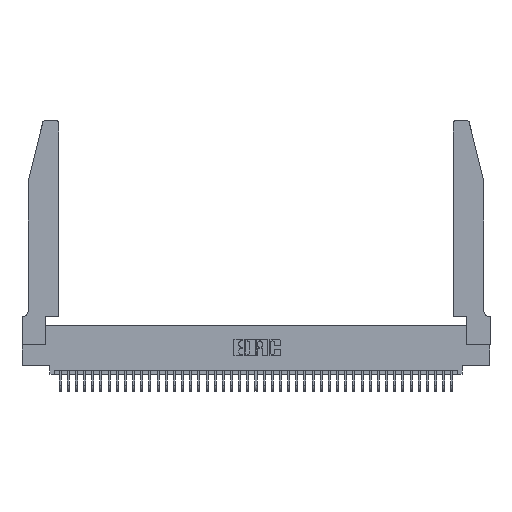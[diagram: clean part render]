
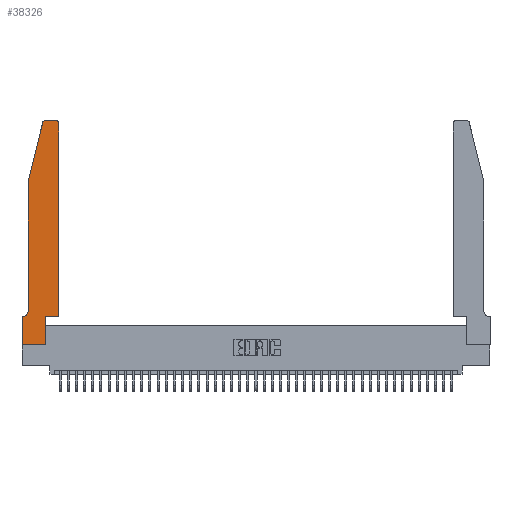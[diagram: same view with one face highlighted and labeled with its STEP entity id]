
A CAD part, top view. The second image highlights one B-rep face of the part: STEP entity #38326.
In plain terms, the highlighted planar face has unit normal (0, 0, 1).
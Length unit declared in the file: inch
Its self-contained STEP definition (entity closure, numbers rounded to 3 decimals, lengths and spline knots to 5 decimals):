
#499 = CARTESIAN_POINT ( 'NONE',  ( 0.0755, 2., 0.37 ) ) ;
#517 = ORIENTED_EDGE ( 'NONE', *, *, #40792, .T. ) ;
#710 = CARTESIAN_POINT ( 'NONE',  ( 0., 0., 0.37 ) ) ;
#1684 = DIRECTION ( 'NONE',  ( -1., 0., 0. ) ) ;
#2917 = DIRECTION ( 'NONE',  ( 0., 0., 1. ) ) ;
#3287 = ORIENTED_EDGE ( 'NONE', *, *, #14220, .T. ) ;
#3686 = EDGE_LOOP ( 'NONE', ( #32409, #3287, #17479, #41431, #13650, #40261, #14280, #517, #28158, #6649, #18911, #6212 ) ) ;
#3842 = DIRECTION ( 'NONE',  ( 1., 0., 0. ) ) ;
#5284 = DIRECTION ( 'NONE',  ( 0., 1., 0. ) ) ;
#5903 = DIRECTION ( 'NONE',  ( 1., 0., 0. ) ) ;
#6018 = CARTESIAN_POINT ( 'NONE',  ( 0.0055, 0.35, 0.37 ) ) ;
#6061 = LINE ( 'NONE', #29420, #16135 ) ;
#6212 = ORIENTED_EDGE ( 'NONE', *, *, #42006, .T. ) ;
#6551 = LINE ( 'NONE', #43830, #17145 ) ;
#6649 = ORIENTED_EDGE ( 'NONE', *, *, #24339, .T. ) ;
#7340 = VERTEX_POINT ( 'NONE', #499 ) ;
#8129 = DIRECTION ( 'NONE',  ( -0.239, -0.971, 0. ) ) ;
#8304 = CARTESIAN_POINT ( 'NONE',  ( 0.0055, 0.42, 0.37 ) ) ;
#8893 = DIRECTION ( 'NONE',  ( 0., -1., 0. ) ) ;
#9343 = CARTESIAN_POINT ( 'NONE',  ( 0., 0., 0.37 ) ) ;
#9999 = AXIS2_PLACEMENT_3D ( 'NONE', #41451, #17824, #31255 ) ;
#10471 = LINE ( 'NONE', #9343, #42308 ) ;
#11280 = EDGE_CURVE ( 'NONE', #39350, #13255, #10471, .T. ) ;
#11479 = FACE_OUTER_BOUND ( 'NONE', #3686, .T. ) ;
#13255 = VERTEX_POINT ( 'NONE', #710 ) ;
#13650 = ORIENTED_EDGE ( 'NONE', *, *, #29005, .T. ) ;
#14220 = EDGE_CURVE ( 'NONE', #36753, #18155, #42134, .T. ) ;
#14280 = ORIENTED_EDGE ( 'NONE', *, *, #11280, .T. ) ;
#14797 = CARTESIAN_POINT ( 'NONE',  ( 0.284, 2.75, 0.37 ) ) ;
#15051 = LINE ( 'NONE', #43553, #32064 ) ;
#15242 = DIRECTION ( 'NONE',  ( 0., 0., -1. ) ) ;
#15613 = EDGE_CURVE ( 'NONE', #42889, #36007, #6061, .T. ) ;
#16135 = VECTOR ( 'NONE', #5284, 39.37008 ) ;
#16411 = CARTESIAN_POINT ( 'NONE',  ( 0.4505, 0.35, 0.37 ) ) ;
#17145 = VECTOR ( 'NONE', #33601, 39.37008 ) ;
#17454 = LINE ( 'NONE', #43038, #37149 ) ;
#17479 = ORIENTED_EDGE ( 'NONE', *, *, #18498, .T. ) ;
#17507 = CARTESIAN_POINT ( 'NONE',  ( 0.2865, 0., 0.37 ) ) ;
#17824 = DIRECTION ( 'NONE',  ( 0., 0., 1. ) ) ;
#18155 = VERTEX_POINT ( 'NONE', #26859 ) ;
#18498 = EDGE_CURVE ( 'NONE', #18155, #7340, #31305, .T. ) ;
#18834 = CARTESIAN_POINT ( 'NONE',  ( 0.4205, 2.72, 0.37 ) ) ;
#18911 = ORIENTED_EDGE ( 'NONE', *, *, #15613, .T. ) ;
#20234 = VERTEX_POINT ( 'NONE', #27464 ) ;
#20630 = DIRECTION ( 'NONE',  ( 1., 0., 0. ) ) ;
#21349 = LINE ( 'NONE', #31890, #43174 ) ;
#21889 = VERTEX_POINT ( 'NONE', #35162 ) ;
#22572 = CARTESIAN_POINT ( 'NONE',  ( 0.0755, 0.35, 0.37 ) ) ;
#23639 = DIRECTION ( 'NONE',  ( 0., 0., 1. ) ) ;
#24339 = EDGE_CURVE ( 'NONE', #21889, #42889, #37945, .T. ) ;
#24898 = EDGE_CURVE ( 'NONE', #20234, #36753, #15051, .T. ) ;
#26571 = AXIS2_PLACEMENT_3D ( 'NONE', #18834, #2917, #36954 ) ;
#26623 = VERTEX_POINT ( 'NONE', #17507 ) ;
#26859 = CARTESIAN_POINT ( 'NONE',  ( 0.25487, 2.72718, 0.37 ) ) ;
#27119 = VECTOR ( 'NONE', #8129, 39.37008 ) ;
#27448 = EDGE_CURVE ( 'NONE', #31205, #39350, #36684, .T. ) ;
#27464 = CARTESIAN_POINT ( 'NONE',  ( 0.4205, 2.75, 0.37 ) ) ;
#28016 = EDGE_CURVE ( 'NONE', #7340, #35905, #21349, .T. ) ;
#28158 = ORIENTED_EDGE ( 'NONE', *, *, #39593, .T. ) ;
#29005 = EDGE_CURVE ( 'NONE', #35905, #31205, #33258, .T. ) ;
#29420 = CARTESIAN_POINT ( 'NONE',  ( 0.4505, 0.35, 0.37 ) ) ;
#30227 = DIRECTION ( 'NONE',  ( -1., 0., 0. ) ) ;
#31205 = VERTEX_POINT ( 'NONE', #6018 ) ;
#31255 = DIRECTION ( 'NONE',  ( 1., 0., 0. ) ) ;
#31305 = LINE ( 'NONE', #39188, #27119 ) ;
#31890 = CARTESIAN_POINT ( 'NONE',  ( 0.0755, 2., 0.37 ) ) ;
#31963 = CARTESIAN_POINT ( 'NONE',  ( 0.4505, 2.72, 0.37 ) ) ;
#31996 = CARTESIAN_POINT ( 'NONE',  ( 0., 0.35, 0.37 ) ) ;
#32064 = VECTOR ( 'NONE', #30227, 39.37008 ) ;
#32409 = ORIENTED_EDGE ( 'NONE', *, *, #24898, .T. ) ;
#33258 = CIRCLE ( 'NONE', #38742, 0.07 ) ;
#33601 = DIRECTION ( 'NONE',  ( 0., 1., 0. ) ) ;
#34276 = PLANE ( 'NONE',  #43488 ) ;
#34323 = CARTESIAN_POINT ( 'NONE',  ( 0.4505, 0.35, 0.37 ) ) ;
#34508 = CIRCLE ( 'NONE', #26571, 0.03 ) ;
#35162 = CARTESIAN_POINT ( 'NONE',  ( 0.2865, 0.35, 0.37 ) ) ;
#35905 = VERTEX_POINT ( 'NONE', #41267 ) ;
#36007 = VERTEX_POINT ( 'NONE', #31963 ) ;
#36684 = LINE ( 'NONE', #22572, #38778 ) ;
#36753 = VERTEX_POINT ( 'NONE', #14797 ) ;
#36954 = DIRECTION ( 'NONE',  ( 1., 0., 0. ) ) ;
#37149 = VECTOR ( 'NONE', #5903, 39.37008 ) ;
#37945 = LINE ( 'NONE', #34323, #41653 ) ;
#37950 = DIRECTION ( 'NONE',  ( 0., -1., 0. ) ) ;
#38326 = ADVANCED_FACE ( 'NONE', ( #11479 ), #34276, .T. ) ;
#38742 = AXIS2_PLACEMENT_3D ( 'NONE', #8304, #15242, #42449 ) ;
#38778 = VECTOR ( 'NONE', #1684, 39.37008 ) ;
#39188 = CARTESIAN_POINT ( 'NONE',  ( 0.0755, 2., 0.37 ) ) ;
#39350 = VERTEX_POINT ( 'NONE', #31996 ) ;
#39593 = EDGE_CURVE ( 'NONE', #26623, #21889, #6551, .T. ) ;
#40261 = ORIENTED_EDGE ( 'NONE', *, *, #27448, .T. ) ;
#40792 = EDGE_CURVE ( 'NONE', #13255, #26623, #17454, .T. ) ;
#41267 = CARTESIAN_POINT ( 'NONE',  ( 0.0755, 0.42, 0.37 ) ) ;
#41431 = ORIENTED_EDGE ( 'NONE', *, *, #28016, .T. ) ;
#41451 = CARTESIAN_POINT ( 'NONE',  ( 0.284, 2.72, 0.37 ) ) ;
#41653 = VECTOR ( 'NONE', #3842, 39.37008 ) ;
#42006 = EDGE_CURVE ( 'NONE', #36007, #20234, #34508, .T. ) ;
#42134 = CIRCLE ( 'NONE', #9999, 0.03 ) ;
#42308 = VECTOR ( 'NONE', #8893, 39.37008 ) ;
#42449 = DIRECTION ( 'NONE',  ( -1., 0., 0. ) ) ;
#42889 = VERTEX_POINT ( 'NONE', #16411 ) ;
#42992 = CARTESIAN_POINT ( 'NONE',  ( 0., 0.35, 0.37 ) ) ;
#43038 = CARTESIAN_POINT ( 'NONE',  ( 0., 0., 0.37 ) ) ;
#43174 = VECTOR ( 'NONE', #37950, 39.37008 ) ;
#43488 = AXIS2_PLACEMENT_3D ( 'NONE', #42992, #23639, #20630 ) ;
#43553 = CARTESIAN_POINT ( 'NONE',  ( 0.2605, 2.75, 0.37 ) ) ;
#43830 = CARTESIAN_POINT ( 'NONE',  ( 0.2865, 0.35, 0.37 ) ) ;
